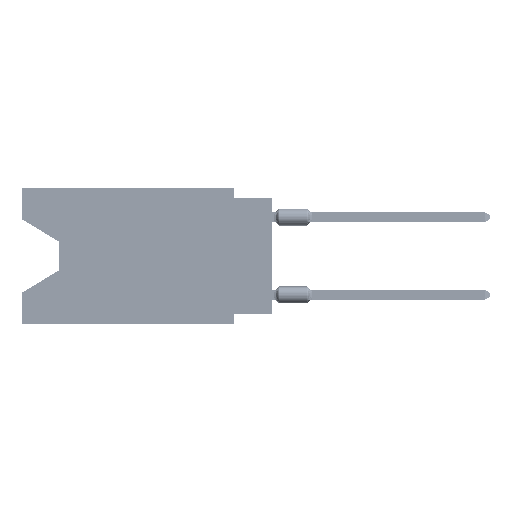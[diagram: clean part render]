
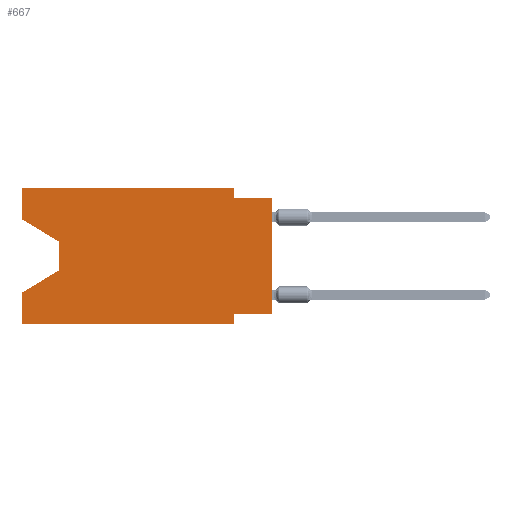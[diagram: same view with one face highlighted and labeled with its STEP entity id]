
A CAD part, left-side view. The second image highlights one B-rep face of the part: STEP entity #667.
In plain terms, the highlighted planar face has unit normal (-1, 0, 0).
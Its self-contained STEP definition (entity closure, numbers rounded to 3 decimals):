
#667 = ADVANCED_FACE ( 'NONE', ( #63132 ), #28327, .F. ) ;
#747 = DIRECTION ( 'NONE',  ( 0., -0.855, -0.519 ) ) ;
#1277 = ORIENTED_EDGE ( 'NONE', *, *, #9406, .T. ) ;
#5240 = ORIENTED_EDGE ( 'NONE', *, *, #67165, .F. ) ;
#6615 = EDGE_CURVE ( 'NONE', #90701, #48075, #35616, .T. ) ;
#9120 = CARTESIAN_POINT ( 'NONE',  ( 0., 0., -0.635 ) ) ;
#9406 = EDGE_CURVE ( 'NONE', #90701, #85917, #77634, .T. ) ;
#10023 = CARTESIAN_POINT ( 'NONE',  ( 0., 2.54, -8.89 ) ) ;
#11666 = DIRECTION ( 'NONE',  ( 0., 0., -1. ) ) ;
#14115 = VERTEX_POINT ( 'NONE', #72194 ) ;
#16856 = VECTOR ( 'NONE', #17025, 1000. ) ;
#17025 = DIRECTION ( 'NONE',  ( 0., 0., 1. ) ) ;
#17761 = CARTESIAN_POINT ( 'NONE',  ( 0., 0., -8.255 ) ) ;
#18098 = VERTEX_POINT ( 'NONE', #99788 ) ;
#18125 = CARTESIAN_POINT ( 'NONE',  ( 0., 16.383, 0. ) ) ;
#18286 = VECTOR ( 'NONE', #42995, 1000. ) ;
#18993 = EDGE_CURVE ( 'NONE', #81365, #30317, #59101, .T. ) ;
#19404 = LINE ( 'NONE', #17761, #18286 ) ;
#20230 = EDGE_CURVE ( 'NONE', #40766, #64717, #93923, .T. ) ;
#20558 = CARTESIAN_POINT ( 'NONE',  ( 0., 16.383, 0. ) ) ;
#22983 = VERTEX_POINT ( 'NONE', #98465 ) ;
#28327 = PLANE ( 'NONE',  #59642 ) ;
#28516 = LINE ( 'NONE', #96443, #91105 ) ;
#29135 = EDGE_CURVE ( 'NONE', #78872, #30317, #36899, .T. ) ;
#29899 = CARTESIAN_POINT ( 'NONE',  ( 0., 0., -8.255 ) ) ;
#30317 = VERTEX_POINT ( 'NONE', #10023 ) ;
#32248 = DIRECTION ( 'NONE',  ( 0., 0., -1. ) ) ;
#34252 = EDGE_CURVE ( 'NONE', #81365, #18098, #55864, .T. ) ;
#34932 = CARTESIAN_POINT ( 'NONE',  ( 0., 16.383, -8.89 ) ) ;
#35069 = CARTESIAN_POINT ( 'NONE',  ( 0., 16.383, 0. ) ) ;
#35616 = LINE ( 'NONE', #35069, #42065 ) ;
#36899 = LINE ( 'NONE', #80663, #106114 ) ;
#39532 = ORIENTED_EDGE ( 'NONE', *, *, #103244, .F. ) ;
#40588 = EDGE_CURVE ( 'NONE', #85917, #14115, #108590, .T. ) ;
#40766 = VERTEX_POINT ( 'NONE', #29899 ) ;
#41015 = VECTOR ( 'NONE', #43363, 1000. ) ;
#41222 = ORIENTED_EDGE ( 'NONE', *, *, #29135, .F. ) ;
#42065 = VECTOR ( 'NONE', #77732, 1000. ) ;
#42995 = DIRECTION ( 'NONE',  ( 0., 1., 0. ) ) ;
#43363 = DIRECTION ( 'NONE',  ( 0., -1., 0. ) ) ;
#46259 = DIRECTION ( 'NONE',  ( 1., 0., 0. ) ) ;
#47082 = ORIENTED_EDGE ( 'NONE', *, *, #34252, .F. ) ;
#47299 = EDGE_LOOP ( 'NONE', ( #1277, #103811, #105224, #47082, #98478, #41222, #5240, #71994, #74705, #88264, #39532, #102944 ) ) ;
#47973 = DIRECTION ( 'NONE',  ( 0., 0., 1. ) ) ;
#48075 = VERTEX_POINT ( 'NONE', #52746 ) ;
#48386 = VERTEX_POINT ( 'NONE', #75668 ) ;
#52514 = CARTESIAN_POINT ( 'NONE',  ( 0., 16.383, -2.038 ) ) ;
#52746 = CARTESIAN_POINT ( 'NONE',  ( 0., 16.383, 0. ) ) ;
#53274 = VECTOR ( 'NONE', #47973, 1000. ) ;
#55864 = LINE ( 'NONE', #20558, #53274 ) ;
#58606 = CARTESIAN_POINT ( 'NONE',  ( 0., 13.97, -5.385 ) ) ;
#59101 = LINE ( 'NONE', #34932, #68696 ) ;
#59642 = AXIS2_PLACEMENT_3D ( 'NONE', #62573, #46259, #95711 ) ;
#59930 = CARTESIAN_POINT ( 'NONE',  ( 0., 2.54, -8.255 ) ) ;
#62573 = CARTESIAN_POINT ( 'NONE',  ( 0., 16.383, 0. ) ) ;
#63132 = FACE_OUTER_BOUND ( 'NONE', #47299, .T. ) ;
#64717 = VERTEX_POINT ( 'NONE', #9120 ) ;
#66724 = CARTESIAN_POINT ( 'NONE',  ( 0., 16.383, -8.89 ) ) ;
#67039 = LINE ( 'NONE', #58606, #95374 ) ;
#67165 = EDGE_CURVE ( 'NONE', #40766, #78872, #19404, .T. ) ;
#67598 = EDGE_CURVE ( 'NONE', #14115, #18098, #67039, .T. ) ;
#68696 = VECTOR ( 'NONE', #86023, 1000. ) ;
#71994 = ORIENTED_EDGE ( 'NONE', *, *, #20230, .T. ) ;
#72194 = CARTESIAN_POINT ( 'NONE',  ( 0., 13.97, -5.385 ) ) ;
#74705 = ORIENTED_EDGE ( 'NONE', *, *, #80117, .F. ) ;
#75668 = CARTESIAN_POINT ( 'NONE',  ( 0., 2.54, 0. ) ) ;
#77611 = LINE ( 'NONE', #18125, #41015 ) ;
#77634 = LINE ( 'NONE', #110758, #96233 ) ;
#77732 = DIRECTION ( 'NONE',  ( 0., 0., 1. ) ) ;
#78872 = VERTEX_POINT ( 'NONE', #59930 ) ;
#79627 = VECTOR ( 'NONE', #100924, 1000. ) ;
#80117 = EDGE_CURVE ( 'NONE', #22983, #64717, #83529, .T. ) ;
#80663 = CARTESIAN_POINT ( 'NONE',  ( 0., 2.54, -8.89 ) ) ;
#81365 = VERTEX_POINT ( 'NONE', #66724 ) ;
#83529 = LINE ( 'NONE', #107116, #79627 ) ;
#85917 = VERTEX_POINT ( 'NONE', #107746 ) ;
#86023 = DIRECTION ( 'NONE',  ( 0., -1., 0. ) ) ;
#88264 = ORIENTED_EDGE ( 'NONE', *, *, #110872, .F. ) ;
#90701 = VERTEX_POINT ( 'NONE', #52514 ) ;
#91105 = VECTOR ( 'NONE', #95901, 1000. ) ;
#92854 = DIRECTION ( 'NONE',  ( 0., 0.855, -0.519 ) ) ;
#93923 = LINE ( 'NONE', #102313, #16856 ) ;
#95374 = VECTOR ( 'NONE', #92854, 1000. ) ;
#95711 = DIRECTION ( 'NONE',  ( 0., 0., -1. ) ) ;
#95901 = DIRECTION ( 'NONE',  ( 0., 0., -1. ) ) ;
#96233 = VECTOR ( 'NONE', #747, 1000. ) ;
#96443 = CARTESIAN_POINT ( 'NONE',  ( 0., 2.54, 0. ) ) ;
#98465 = CARTESIAN_POINT ( 'NONE',  ( 0., 2.54, -0.635 ) ) ;
#98478 = ORIENTED_EDGE ( 'NONE', *, *, #18993, .T. ) ;
#99788 = CARTESIAN_POINT ( 'NONE',  ( 0., 16.383, -6.852 ) ) ;
#100924 = DIRECTION ( 'NONE',  ( 0., -1., 0. ) ) ;
#102313 = CARTESIAN_POINT ( 'NONE',  ( 0., 0., 0. ) ) ;
#102944 = ORIENTED_EDGE ( 'NONE', *, *, #6615, .F. ) ;
#103244 = EDGE_CURVE ( 'NONE', #48075, #48386, #77611, .T. ) ;
#103811 = ORIENTED_EDGE ( 'NONE', *, *, #40588, .T. ) ;
#104490 = VECTOR ( 'NONE', #32248, 1000. ) ;
#105224 = ORIENTED_EDGE ( 'NONE', *, *, #67598, .T. ) ;
#106114 = VECTOR ( 'NONE', #11666, 1000. ) ;
#107116 = CARTESIAN_POINT ( 'NONE',  ( 0., 0., -0.635 ) ) ;
#107746 = CARTESIAN_POINT ( 'NONE',  ( 0., 13.97, -3.505 ) ) ;
#108590 = LINE ( 'NONE', #109141, #104490 ) ;
#109141 = CARTESIAN_POINT ( 'NONE',  ( 0., 13.97, -3.505 ) ) ;
#110758 = CARTESIAN_POINT ( 'NONE',  ( 0., 16.383, -2.038 ) ) ;
#110872 = EDGE_CURVE ( 'NONE', #48386, #22983, #28516, .T. ) ;
